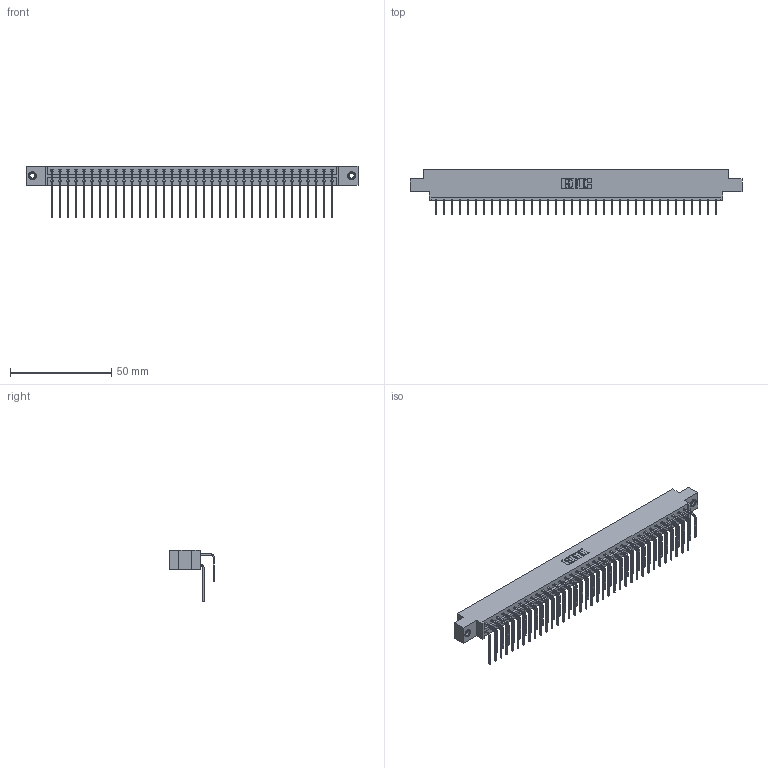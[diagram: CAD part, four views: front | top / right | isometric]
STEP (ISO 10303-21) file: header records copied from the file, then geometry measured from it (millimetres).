
FILE_DESCRIPTION (( 'STEP AP203' ), '1' );
FILE_NAME ('333-072-558-807.STEP', '2018-08-04T21:14:47', ( '' ), ( '' ), 'SwSTEP 2.0', 'SolidWorks 2016', '' );
FILE_SCHEMA (( 'CONFIG_CONTROL_DESIGN' ));
Length unit declared in the file: inch
Products named in the file (5): 345-292-001_558 Tail - 2; 345-250-001_345-250-005-103; 333-072-558-807; 333 Part_Offset - .156 Dia - TI; 345-292-001_558 559 Tail - 1
Assembly tree (75 placements, depth 2):
  333-072-558-807
    333 Part_Offset - .156 Dia - TI
    345-292-001_558 559 Tail - 1  x36
    345-292-001_558 Tail - 2  x36
    345-250-001_345-250-005-103  x2
Bounding box: 164.19 x 22.17 x 25.53 mm (x, y, z)
Volume: 16880.3 mm3; surface area: 22216.1 mm2
Topology: 75 solids, 75 shells, 4066 faces, 12051 edges, 7930 vertices
Faces by surface type: plane 2842, cylinder 1208, cone 12, torus 4
Entity records: 27038 total; most frequent: CARTESIAN_POINT 4524, ORIENTED_EDGE 4402, DIRECTION 3887, EDGE_CURVE 2201, VECTOR 2013, LINE 2013, VERTEX_POINT 1460, AXIS2_PLACEMENT_3D 937
